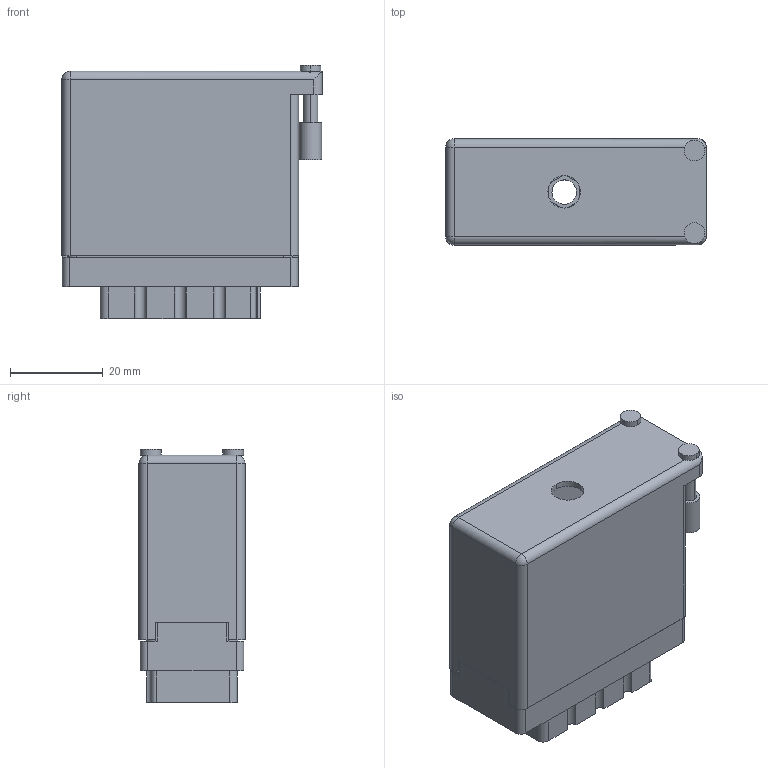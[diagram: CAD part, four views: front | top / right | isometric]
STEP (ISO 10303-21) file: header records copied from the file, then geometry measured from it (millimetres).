
FILE_DESCRIPTION (( 'STEP AP203' ), '1' );
FILE_NAME ('516-038-501-650.STEP', '2020-09-08T15:52:14', ( '' ), ( '' ), 'SwSTEP 2.0', 'SolidWorks 2020', '' );
FILE_SCHEMA (( 'CONFIG_CONTROL_DESIGN' ));
Length unit declared in the file: inch
Products named in the file (4): 516-230-001_Metal - 038 Side Entry; 516-292-001_501 Contact; 516 Part Receptacle_038; 516-038-501-650
Assembly tree (41 placements, depth 2):
  516-038-501-650
    516 Part Receptacle_038
    516-292-001_501 Contact  x39
    516-230-001_Metal - 038 Side Entry
Bounding box: 56.08 x 22.83 x 54.53 mm (x, y, z)
Volume: 20953.7 mm3; surface area: 35278.5 mm2
Topology: 41 solids, 41 shells, 3787 faces, 10975 edges, 7284 vertices
Faces by surface type: plane 2269, cylinder 1280, bspline 234, cone 2, sphere 2
Entity records: 36875 total; most frequent: CARTESIAN_POINT 6530, ORIENTED_EDGE 6138, DIRECTION 6010, EDGE_CURVE 3069, VECTOR 2228, LINE 2228, VERTEX_POINT 2040, AXIS2_PLACEMENT_3D 1891
